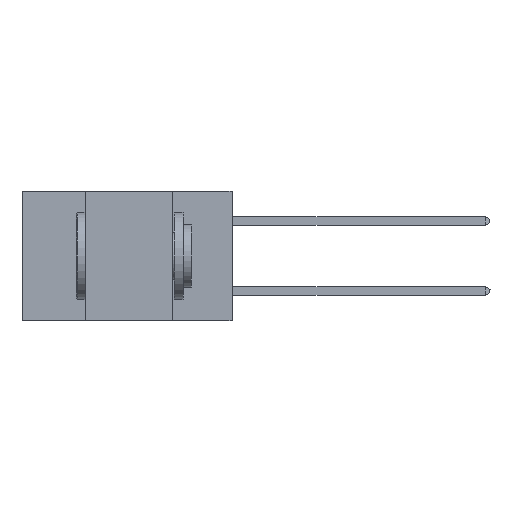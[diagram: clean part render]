
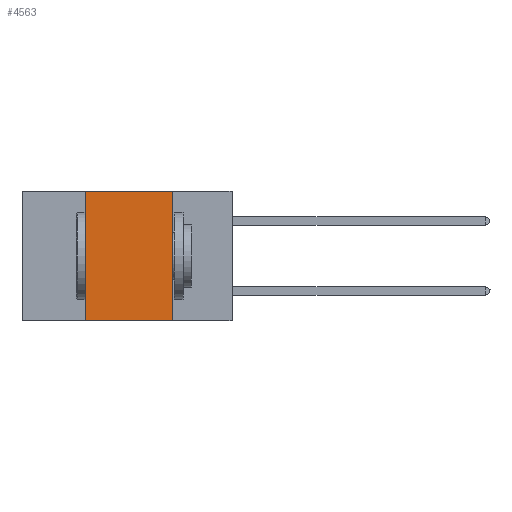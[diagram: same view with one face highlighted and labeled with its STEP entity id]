
A CAD part, left-side view. The second image highlights one B-rep face of the part: STEP entity #4563.
In plain terms, the highlighted planar face has unit normal (-1, 0, 0).
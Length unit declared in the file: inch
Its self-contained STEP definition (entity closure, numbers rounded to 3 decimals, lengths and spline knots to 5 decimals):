
#391 = LINE ( 'NONE', #17839, #10661 ) ;
#414 = AXIS2_PLACEMENT_3D ( 'NONE', #8178, #14618, #17158 ) ;
#539 = LINE ( 'NONE', #10205, #6155 ) ;
#815 = VERTEX_POINT ( 'NONE', #14858 ) ;
#898 = LINE ( 'NONE', #981, #16909 ) ;
#981 = CARTESIAN_POINT ( 'NONE',  ( 0., 0.17, 0. ) ) ;
#1151 = ORIENTED_EDGE ( 'NONE', *, *, #2495, .F. ) ;
#2224 = DIRECTION ( 'NONE',  ( 0., -1., 0. ) ) ;
#2265 = CARTESIAN_POINT ( 'NONE',  ( 0., 0.42, 0. ) ) ;
#2495 = EDGE_CURVE ( 'NONE', #815, #19941, #898, .T. ) ;
#4563 = ADVANCED_FACE ( 'NONE', ( #6186 ), #12564, .F. ) ;
#5511 = VERTEX_POINT ( 'NONE', #14733 ) ;
#6155 = VECTOR ( 'NONE', #2224, 39.37008 ) ;
#6186 = FACE_OUTER_BOUND ( 'NONE', #8088, .T. ) ;
#6773 = DIRECTION ( 'NONE',  ( 0., 0., 1. ) ) ;
#7561 = VECTOR ( 'NONE', #6773, 39.37008 ) ;
#8088 = EDGE_LOOP ( 'NONE', ( #1151, #15153, #10186, #10084 ) ) ;
#8178 = CARTESIAN_POINT ( 'NONE',  ( 0., 0.6, 0. ) ) ;
#8718 = CARTESIAN_POINT ( 'NONE',  ( 0., 0.42, -0.37 ) ) ;
#10084 = ORIENTED_EDGE ( 'NONE', *, *, #12131, .T. ) ;
#10186 = ORIENTED_EDGE ( 'NONE', *, *, #13762, .F. ) ;
#10205 = CARTESIAN_POINT ( 'NONE',  ( 0., 0.6, -0.37 ) ) ;
#10661 = VECTOR ( 'NONE', #13436, 39.37008 ) ;
#10696 = VERTEX_POINT ( 'NONE', #8718 ) ;
#12131 = EDGE_CURVE ( 'NONE', #10696, #19941, #539, .T. ) ;
#12564 = PLANE ( 'NONE',  #414 ) ;
#13436 = DIRECTION ( 'NONE',  ( 0., -1., 0. ) ) ;
#13564 = DIRECTION ( 'NONE',  ( 0., 0., -1. ) ) ;
#13762 = EDGE_CURVE ( 'NONE', #10696, #5511, #19227, .T. ) ;
#14618 = DIRECTION ( 'NONE',  ( 1., 0., 0. ) ) ;
#14733 = CARTESIAN_POINT ( 'NONE',  ( 0., 0.42, 0. ) ) ;
#14858 = CARTESIAN_POINT ( 'NONE',  ( 0., 0.17, 0. ) ) ;
#15153 = ORIENTED_EDGE ( 'NONE', *, *, #15657, .F. ) ;
#15657 = EDGE_CURVE ( 'NONE', #5511, #815, #391, .T. ) ;
#16909 = VECTOR ( 'NONE', #13564, 39.37008 ) ;
#17158 = DIRECTION ( 'NONE',  ( 0., 0., -1. ) ) ;
#17839 = CARTESIAN_POINT ( 'NONE',  ( 0., 0.6, 0. ) ) ;
#19227 = LINE ( 'NONE', #2265, #7561 ) ;
#19738 = CARTESIAN_POINT ( 'NONE',  ( 0., 0.17, -0.37 ) ) ;
#19941 = VERTEX_POINT ( 'NONE', #19738 ) ;
